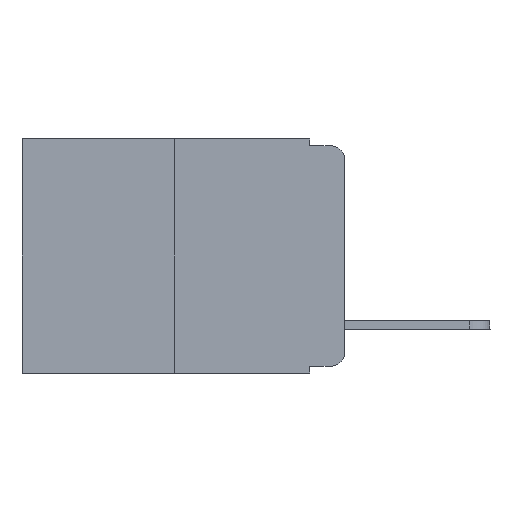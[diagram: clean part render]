
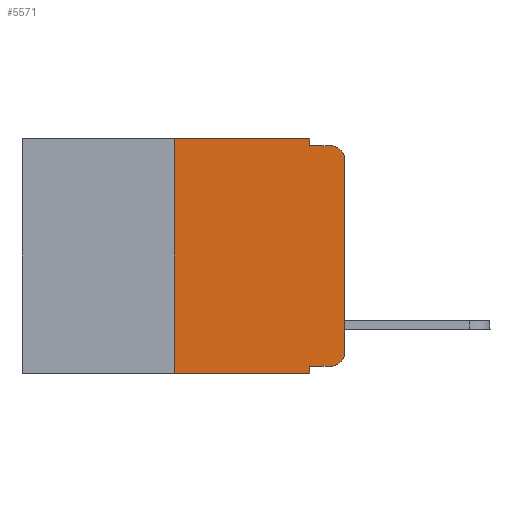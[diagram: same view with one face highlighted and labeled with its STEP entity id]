
A CAD part, left-side view. The second image highlights one B-rep face of the part: STEP entity #5571.
In plain terms, the highlighted planar face has unit normal (-1, 0, 0).
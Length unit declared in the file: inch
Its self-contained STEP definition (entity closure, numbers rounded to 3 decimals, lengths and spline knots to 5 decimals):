
#127 = CARTESIAN_POINT ( 'NONE',  ( 0., 0.25, 0. ) ) ;
#204 = CARTESIAN_POINT ( 'NONE',  ( 0., 0.473, -0.343 ) ) ;
#596 = VECTOR ( 'NONE', #11613, 39.37008 ) ;
#762 = CARTESIAN_POINT ( 'NONE',  ( 0., 0., -0.03 ) ) ;
#765 = VERTEX_POINT ( 'NONE', #2384 ) ;
#844 = CIRCLE ( 'NONE', #2831, 0.02 ) ;
#961 = LINE ( 'NONE', #1835, #4319 ) ;
#988 = ORIENTED_EDGE ( 'NONE', *, *, #8878, .F. ) ;
#1538 = ORIENTED_EDGE ( 'NONE', *, *, #13641, .F. ) ;
#1597 = VECTOR ( 'NONE', #11875, 39.37008 ) ;
#1636 = EDGE_CURVE ( 'NONE', #8891, #11277, #9558, .T. ) ;
#1780 = ORIENTED_EDGE ( 'NONE', *, *, #8810, .T. ) ;
#1835 = CARTESIAN_POINT ( 'NONE',  ( 0., 0.051, -0.333 ) ) ;
#1964 = DIRECTION ( 'NONE',  ( -1., 0., 0. ) ) ;
#1979 = DIRECTION ( 'NONE',  ( 0., -1., 0. ) ) ;
#2384 = CARTESIAN_POINT ( 'NONE',  ( 0., 0.02, -0.333 ) ) ;
#2598 = CARTESIAN_POINT ( 'NONE',  ( 0., 0.051, -0.333 ) ) ;
#2831 = AXIS2_PLACEMENT_3D ( 'NONE', #12708, #1964, #9124 ) ;
#3124 = FACE_OUTER_BOUND ( 'NONE', #5710, .T. ) ;
#3195 = DIRECTION ( 'NONE',  ( 0., 0., -1. ) ) ;
#3735 = CARTESIAN_POINT ( 'NONE',  ( 0., 0.25, 0. ) ) ;
#3910 = ORIENTED_EDGE ( 'NONE', *, *, #8600, .F. ) ;
#4056 = DIRECTION ( 'NONE',  ( 0., 0., -1. ) ) ;
#4180 = EDGE_CURVE ( 'NONE', #765, #14482, #7982, .T. ) ;
#4319 = VECTOR ( 'NONE', #1979, 39.37008 ) ;
#4721 = LINE ( 'NONE', #13279, #14333 ) ;
#4852 = LINE ( 'NONE', #204, #8342 ) ;
#4997 = DIRECTION ( 'NONE',  ( 0., -1., 0. ) ) ;
#5052 = ORIENTED_EDGE ( 'NONE', *, *, #5644, .T. ) ;
#5454 = CARTESIAN_POINT ( 'NONE',  ( 0., 0.02, -0.01 ) ) ;
#5571 = ADVANCED_FACE ( 'NONE', ( #3124 ), #11823, .F. ) ;
#5644 = EDGE_CURVE ( 'NONE', #8891, #14424, #4852, .T. ) ;
#5710 = EDGE_LOOP ( 'NONE', ( #5718, #1780, #3910, #9365, #1538, #8952, #5052, #988, #13800, #14149 ) ) ;
#5718 = ORIENTED_EDGE ( 'NONE', *, *, #14739, .T. ) ;
#5783 = EDGE_CURVE ( 'NONE', #12866, #10058, #8919, .T. ) ;
#5859 = CARTESIAN_POINT ( 'NONE',  ( 0., 0.051, -0.01 ) ) ;
#5880 = CARTESIAN_POINT ( 'NONE',  ( 0., 0.473, 0. ) ) ;
#6929 = CARTESIAN_POINT ( 'NONE',  ( 0., 0.25, -0.343 ) ) ;
#6973 = DIRECTION ( 'NONE',  ( -1., 0., 0. ) ) ;
#7014 = VECTOR ( 'NONE', #4056, 39.37008 ) ;
#7028 = VERTEX_POINT ( 'NONE', #2598 ) ;
#7035 = LINE ( 'NONE', #5859, #1597 ) ;
#7982 = CIRCLE ( 'NONE', #8485, 0.02 ) ;
#8342 = VECTOR ( 'NONE', #4997, 39.37008 ) ;
#8359 = VECTOR ( 'NONE', #15435, 39.37008 ) ;
#8382 = VERTEX_POINT ( 'NONE', #762 ) ;
#8485 = AXIS2_PLACEMENT_3D ( 'NONE', #11506, #6973, #3195 ) ;
#8600 = EDGE_CURVE ( 'NONE', #10058, #14218, #7035, .T. ) ;
#8810 = EDGE_CURVE ( 'NONE', #8382, #14218, #844, .T. ) ;
#8878 = EDGE_CURVE ( 'NONE', #7028, #14424, #12884, .T. ) ;
#8891 = VERTEX_POINT ( 'NONE', #6929 ) ;
#8919 = LINE ( 'NONE', #14661, #7014 ) ;
#8952 = ORIENTED_EDGE ( 'NONE', *, *, #1636, .F. ) ;
#9124 = DIRECTION ( 'NONE',  ( 0., 0., -1. ) ) ;
#9356 = AXIS2_PLACEMENT_3D ( 'NONE', #5880, #10344, #15442 ) ;
#9365 = ORIENTED_EDGE ( 'NONE', *, *, #5783, .F. ) ;
#9476 = CARTESIAN_POINT ( 'NONE',  ( 0., 0.051, 0. ) ) ;
#9558 = LINE ( 'NONE', #127, #8359 ) ;
#9633 = CARTESIAN_POINT ( 'NONE',  ( 0., 0.051, -0.01 ) ) ;
#10058 = VERTEX_POINT ( 'NONE', #9633 ) ;
#10296 = CARTESIAN_POINT ( 'NONE',  ( 0., 0., 0. ) ) ;
#10344 = DIRECTION ( 'NONE',  ( 1., 0., 0. ) ) ;
#10620 = CARTESIAN_POINT ( 'NONE',  ( 0., 0., -0.313 ) ) ;
#11277 = VERTEX_POINT ( 'NONE', #3735 ) ;
#11506 = CARTESIAN_POINT ( 'NONE',  ( 0., 0.02, -0.313 ) ) ;
#11613 = DIRECTION ( 'NONE',  ( 0., 0., -1. ) ) ;
#11823 = PLANE ( 'NONE',  #9356 ) ;
#11875 = DIRECTION ( 'NONE',  ( 0., -1., 0. ) ) ;
#12645 = LINE ( 'NONE', #10296, #13093 ) ;
#12708 = CARTESIAN_POINT ( 'NONE',  ( 0., 0.02, -0.03 ) ) ;
#12798 = CARTESIAN_POINT ( 'NONE',  ( 0., 0.051, 0. ) ) ;
#12866 = VERTEX_POINT ( 'NONE', #9476 ) ;
#12884 = LINE ( 'NONE', #12798, #596 ) ;
#13093 = VECTOR ( 'NONE', #15326, 39.37008 ) ;
#13279 = CARTESIAN_POINT ( 'NONE',  ( 0., 0.473, 0. ) ) ;
#13641 = EDGE_CURVE ( 'NONE', #11277, #12866, #4721, .T. ) ;
#13800 = ORIENTED_EDGE ( 'NONE', *, *, #14819, .T. ) ;
#14098 = CARTESIAN_POINT ( 'NONE',  ( 0., 0.051, -0.343 ) ) ;
#14149 = ORIENTED_EDGE ( 'NONE', *, *, #4180, .T. ) ;
#14154 = DIRECTION ( 'NONE',  ( 0., -1., 0. ) ) ;
#14218 = VERTEX_POINT ( 'NONE', #5454 ) ;
#14333 = VECTOR ( 'NONE', #14154, 39.37008 ) ;
#14424 = VERTEX_POINT ( 'NONE', #14098 ) ;
#14482 = VERTEX_POINT ( 'NONE', #10620 ) ;
#14661 = CARTESIAN_POINT ( 'NONE',  ( 0., 0.051, 0. ) ) ;
#14739 = EDGE_CURVE ( 'NONE', #14482, #8382, #12645, .T. ) ;
#14819 = EDGE_CURVE ( 'NONE', #7028, #765, #961, .T. ) ;
#15326 = DIRECTION ( 'NONE',  ( 0., 0., 1. ) ) ;
#15435 = DIRECTION ( 'NONE',  ( 0., 0., 1. ) ) ;
#15442 = DIRECTION ( 'NONE',  ( 0., 0., -1. ) ) ;
